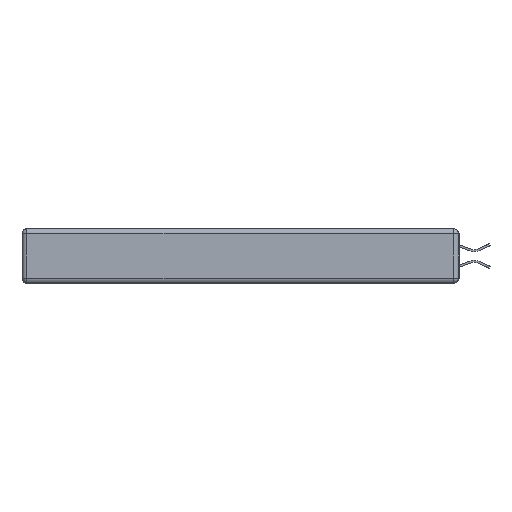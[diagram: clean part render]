
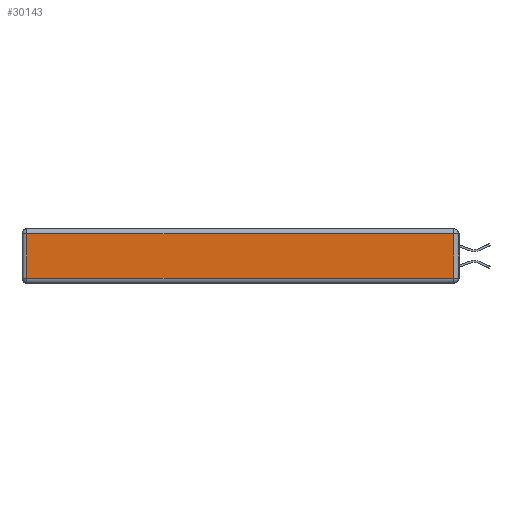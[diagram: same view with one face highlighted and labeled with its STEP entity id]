
A CAD part, left-side view. The second image highlights one B-rep face of the part: STEP entity #30143.
In plain terms, the highlighted planar face has unit normal (-1, 0, 0).
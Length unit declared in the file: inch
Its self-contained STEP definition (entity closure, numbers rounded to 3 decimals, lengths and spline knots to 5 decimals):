
#234 = VERTEX_POINT ( 'NONE', #19794 ) ;
#588 = PLANE ( 'NONE',  #20845 ) ;
#703 = EDGE_CURVE ( 'NONE', #18033, #20885, #12649, .T. ) ;
#2015 = EDGE_LOOP ( 'NONE', ( #8743, #20729, #19874, #26525 ) ) ;
#6626 = EDGE_CURVE ( 'NONE', #20885, #21160, #14258, .T. ) ;
#7129 = VECTOR ( 'NONE', #24561, 39.37008 ) ;
#7151 = LINE ( 'NONE', #24568, #20290 ) ;
#8059 = CARTESIAN_POINT ( 'NONE',  ( 0., 0., -0.313 ) ) ;
#8743 = ORIENTED_EDGE ( 'NONE', *, *, #6626, .T. ) ;
#10908 = DIRECTION ( 'NONE',  ( 0., 0., 1. ) ) ;
#12101 = LINE ( 'NONE', #25232, #29786 ) ;
#12290 = CARTESIAN_POINT ( 'NONE',  ( 0., 2.72, -0.313 ) ) ;
#12649 = LINE ( 'NONE', #17321, #15269 ) ;
#14258 = LINE ( 'NONE', #8059, #7129 ) ;
#14529 = EDGE_CURVE ( 'NONE', #234, #18033, #7151, .T. ) ;
#14679 = DIRECTION ( 'NONE',  ( 0., 0., -1. ) ) ;
#15053 = CARTESIAN_POINT ( 'NONE',  ( 0., 0., -0.343 ) ) ;
#15269 = VECTOR ( 'NONE', #14679, 39.37008 ) ;
#17321 = CARTESIAN_POINT ( 'NONE',  ( 0., 2.72, -0.343 ) ) ;
#17481 = DIRECTION ( 'NONE',  ( 0., 0., 1. ) ) ;
#18033 = VERTEX_POINT ( 'NONE', #19466 ) ;
#19466 = CARTESIAN_POINT ( 'NONE',  ( 0., 2.72, -0.03 ) ) ;
#19794 = CARTESIAN_POINT ( 'NONE',  ( 0., 0.03, -0.03 ) ) ;
#19874 = ORIENTED_EDGE ( 'NONE', *, *, #14529, .T. ) ;
#20290 = VECTOR ( 'NONE', #29281, 39.37008 ) ;
#20482 = FACE_OUTER_BOUND ( 'NONE', #2015, .T. ) ;
#20729 = ORIENTED_EDGE ( 'NONE', *, *, #20737, .T. ) ;
#20737 = EDGE_CURVE ( 'NONE', #21160, #234, #12101, .T. ) ;
#20845 = AXIS2_PLACEMENT_3D ( 'NONE', #15053, #29783, #17481 ) ;
#20885 = VERTEX_POINT ( 'NONE', #12290 ) ;
#21160 = VERTEX_POINT ( 'NONE', #29180 ) ;
#24561 = DIRECTION ( 'NONE',  ( 0., -1., 0. ) ) ;
#24568 = CARTESIAN_POINT ( 'NONE',  ( 0., 2.75, -0.03 ) ) ;
#25232 = CARTESIAN_POINT ( 'NONE',  ( 0., 0.03, -0.343 ) ) ;
#26525 = ORIENTED_EDGE ( 'NONE', *, *, #703, .T. ) ;
#29180 = CARTESIAN_POINT ( 'NONE',  ( 0., 0.03, -0.313 ) ) ;
#29281 = DIRECTION ( 'NONE',  ( 0., 1., 0. ) ) ;
#29783 = DIRECTION ( 'NONE',  ( -1., 0., 0. ) ) ;
#29786 = VECTOR ( 'NONE', #10908, 39.37008 ) ;
#30143 = ADVANCED_FACE ( 'NONE', ( #20482 ), #588, .T. ) ;
